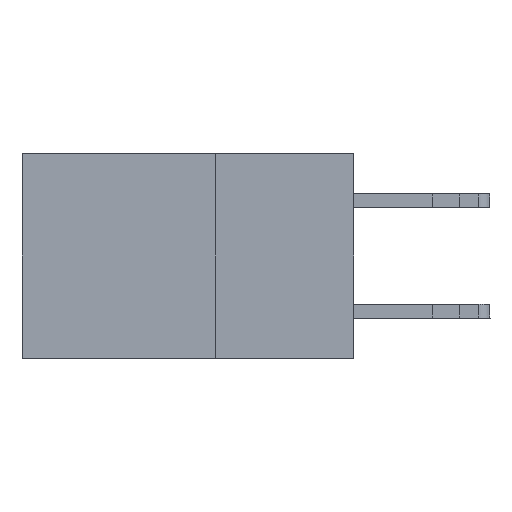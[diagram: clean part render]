
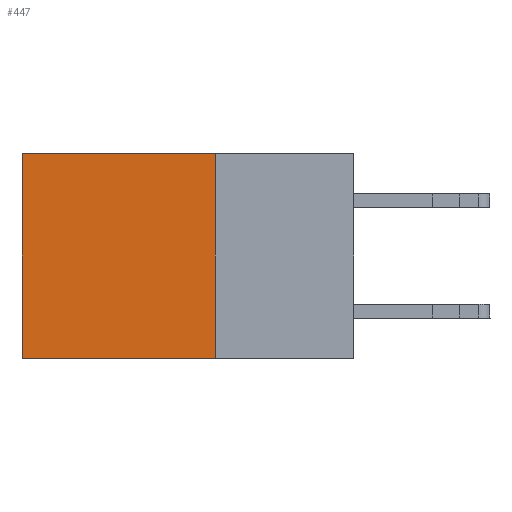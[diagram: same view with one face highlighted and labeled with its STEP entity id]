
A CAD part, left-side view. The second image highlights one B-rep face of the part: STEP entity #447.
In plain terms, the highlighted planar face has unit normal (-1, 0, 0).
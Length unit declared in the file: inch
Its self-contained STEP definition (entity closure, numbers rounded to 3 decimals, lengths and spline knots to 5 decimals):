
#94 = VECTOR ( 'NONE', #3354, 39.37008 ) ;
#107 = CARTESIAN_POINT ( 'NONE',  ( 0.2875, 0.25, 0. ) ) ;
#447 = ADVANCED_FACE ( 'NONE', ( #19969 ), #13993, .F. ) ;
#979 = LINE ( 'NONE', #4717, #14255 ) ;
#1028 = DIRECTION ( 'NONE',  ( 0., 0., -1. ) ) ;
#1112 = VERTEX_POINT ( 'NONE', #4688 ) ;
#1403 = EDGE_CURVE ( 'NONE', #13864, #8421, #14499, .T. ) ;
#1491 = DIRECTION ( 'NONE',  ( 1., 0., 0. ) ) ;
#3354 = DIRECTION ( 'NONE',  ( 0., 0., -1. ) ) ;
#4688 = CARTESIAN_POINT ( 'NONE',  ( 0.2875, 0.25, 0. ) ) ;
#4717 = CARTESIAN_POINT ( 'NONE',  ( 0.2875, 0.25, 0. ) ) ;
#5465 = CARTESIAN_POINT ( 'NONE',  ( 0.2875, 0.6, -0.37 ) ) ;
#5977 = DIRECTION ( 'NONE',  ( 0., 0., -1. ) ) ;
#6728 = CARTESIAN_POINT ( 'NONE',  ( 0.2875, 0.6, 0. ) ) ;
#6779 = ORIENTED_EDGE ( 'NONE', *, *, #13961, .F. ) ;
#7672 = EDGE_LOOP ( 'NONE', ( #14822, #6779, #21549, #21754 ) ) ;
#8421 = VERTEX_POINT ( 'NONE', #5465 ) ;
#8697 = CARTESIAN_POINT ( 'NONE',  ( 0.2875, 0.25, -0.37 ) ) ;
#8732 = AXIS2_PLACEMENT_3D ( 'NONE', #107, #1491, #5977 ) ;
#10147 = CARTESIAN_POINT ( 'NONE',  ( 0.2875, 0.25, 0. ) ) ;
#10719 = VECTOR ( 'NONE', #17516, 39.37008 ) ;
#11851 = VERTEX_POINT ( 'NONE', #16271 ) ;
#13864 = VERTEX_POINT ( 'NONE', #6728 ) ;
#13961 = EDGE_CURVE ( 'NONE', #11851, #8421, #20029, .T. ) ;
#13993 = PLANE ( 'NONE',  #8732 ) ;
#14255 = VECTOR ( 'NONE', #1028, 39.37008 ) ;
#14499 = LINE ( 'NONE', #19213, #94 ) ;
#14742 = LINE ( 'NONE', #10147, #19380 ) ;
#14822 = ORIENTED_EDGE ( 'NONE', *, *, #1403, .T. ) ;
#16271 = CARTESIAN_POINT ( 'NONE',  ( 0.2875, 0.25, -0.37 ) ) ;
#17348 = EDGE_CURVE ( 'NONE', #1112, #11851, #979, .T. ) ;
#17516 = DIRECTION ( 'NONE',  ( 0., 1., 0. ) ) ;
#18675 = EDGE_CURVE ( 'NONE', #1112, #13864, #14742, .T. ) ;
#19213 = CARTESIAN_POINT ( 'NONE',  ( 0.2875, 0.6, 0. ) ) ;
#19380 = VECTOR ( 'NONE', #22365, 39.37008 ) ;
#19969 = FACE_OUTER_BOUND ( 'NONE', #7672, .T. ) ;
#20029 = LINE ( 'NONE', #8697, #10719 ) ;
#21549 = ORIENTED_EDGE ( 'NONE', *, *, #17348, .F. ) ;
#21754 = ORIENTED_EDGE ( 'NONE', *, *, #18675, .T. ) ;
#22365 = DIRECTION ( 'NONE',  ( 0., 1., 0. ) ) ;
